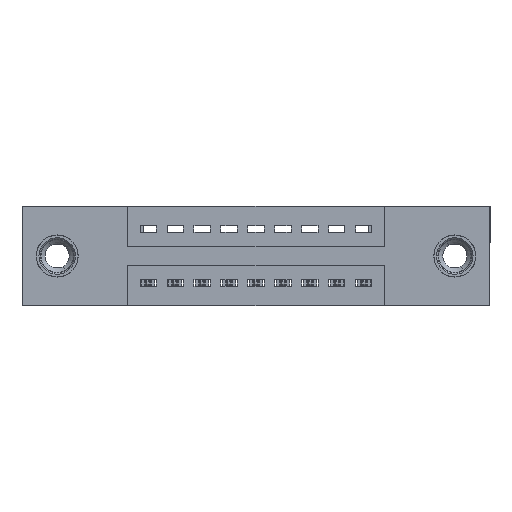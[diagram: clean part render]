
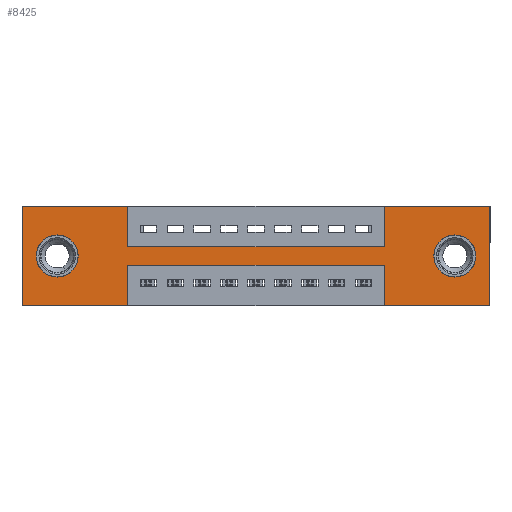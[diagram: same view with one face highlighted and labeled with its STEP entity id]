
A CAD part, front view. The second image highlights one B-rep face of the part: STEP entity #8425.
In plain terms, the highlighted planar face has unit normal (0, -1, 0).
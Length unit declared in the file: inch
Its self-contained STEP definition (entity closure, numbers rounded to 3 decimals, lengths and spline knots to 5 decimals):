
#80 = EDGE_CURVE ( 'NONE', #3752, #586, #3976, .T. ) ;
#113 = EDGE_CURVE ( 'NONE', #8983, #13188, #11638, .T. ) ;
#175 = DIRECTION ( 'NONE',  ( 0., 0., -1. ) ) ;
#392 = DIRECTION ( 'NONE',  ( 0., 1., 0. ) ) ;
#417 = LINE ( 'NONE', #14052, #2769 ) ;
#498 = ORIENTED_EDGE ( 'NONE', *, *, #80, .F. ) ;
#586 = VERTEX_POINT ( 'NONE', #14877 ) ;
#707 = ORIENTED_EDGE ( 'NONE', *, *, #6458, .F. ) ;
#833 = ORIENTED_EDGE ( 'NONE', *, *, #4061, .F. ) ;
#835 = EDGE_CURVE ( 'NONE', #6076, #4176, #8668, .T. ) ;
#995 = VECTOR ( 'NONE', #7859, 39.37008 ) ;
#1015 = VECTOR ( 'NONE', #15629, 39.37008 ) ;
#1167 = VERTEX_POINT ( 'NONE', #13422 ) ;
#1375 = VECTOR ( 'NONE', #2365, 39.37008 ) ;
#1407 = EDGE_CURVE ( 'NONE', #15398, #14669, #15788, .T. ) ;
#1421 = EDGE_CURVE ( 'NONE', #1167, #15398, #10657, .T. ) ;
#1586 = CARTESIAN_POINT ( 'NONE',  ( 0., 0., 0. ) ) ;
#1624 = DIRECTION ( 'NONE',  ( 0., -1., 0. ) ) ;
#1841 = EDGE_CURVE ( 'NONE', #9215, #12019, #5447, .T. ) ;
#1917 = VERTEX_POINT ( 'NONE', #3120 ) ;
#2189 = ORIENTED_EDGE ( 'NONE', *, *, #7108, .F. ) ;
#2365 = DIRECTION ( 'NONE',  ( -1., 0., 0. ) ) ;
#2640 = VECTOR ( 'NONE', #10238, 39.37008 ) ;
#2645 = CARTESIAN_POINT ( 'NONE',  ( 0.3925, 0., -0.37 ) ) ;
#2660 = CARTESIAN_POINT ( 'NONE',  ( 0., 0., -0.37 ) ) ;
#2769 = VECTOR ( 'NONE', #11385, 39.37008 ) ;
#2823 = CARTESIAN_POINT ( 'NONE',  ( 0.13, 0., -0.107 ) ) ;
#2873 = CARTESIAN_POINT ( 'NONE',  ( 1.735, 0., 0. ) ) ;
#2982 = CARTESIAN_POINT ( 'NONE',  ( 1.605, 0., -0.263 ) ) ;
#3120 = CARTESIAN_POINT ( 'NONE',  ( 1.3425, 0., -0.37 ) ) ;
#3184 = CARTESIAN_POINT ( 'NONE',  ( 1.3425, 0., 0. ) ) ;
#3246 = ORIENTED_EDGE ( 'NONE', *, *, #8589, .F. ) ;
#3310 = EDGE_LOOP ( 'NONE', ( #13696, #6005, #3246, #2189, #6740, #5573, #14188, #707, #12571, #498, #7220, #833 ) ) ;
#3475 = EDGE_CURVE ( 'NONE', #12019, #9215, #6502, .T. ) ;
#3740 = VECTOR ( 'NONE', #4452, 39.37008 ) ;
#3752 = VERTEX_POINT ( 'NONE', #6639 ) ;
#3893 = LINE ( 'NONE', #2660, #8349 ) ;
#3976 = LINE ( 'NONE', #1586, #995 ) ;
#4061 = EDGE_CURVE ( 'NONE', #4176, #5098, #3893, .T. ) ;
#4176 = VERTEX_POINT ( 'NONE', #6863 ) ;
#4195 = EDGE_CURVE ( 'NONE', #4606, #6076, #9405, .T. ) ;
#4267 = CARTESIAN_POINT ( 'NONE',  ( 1.605, 0., -0.185 ) ) ;
#4347 = DIRECTION ( 'NONE',  ( 0., 0., -1. ) ) ;
#4418 = DIRECTION ( 'NONE',  ( 0., 1., 0. ) ) ;
#4452 = DIRECTION ( 'NONE',  ( 1., 0., 0. ) ) ;
#4495 = EDGE_CURVE ( 'NONE', #5098, #3752, #7562, .T. ) ;
#4606 = VERTEX_POINT ( 'NONE', #9433 ) ;
#4640 = VECTOR ( 'NONE', #10030, 39.37008 ) ;
#4838 = CARTESIAN_POINT ( 'NONE',  ( 1.735, 0., 0. ) ) ;
#5098 = VERTEX_POINT ( 'NONE', #11167 ) ;
#5101 = AXIS2_PLACEMENT_3D ( 'NONE', #12223, #13770, #7516 ) ;
#5447 = CIRCLE ( 'NONE', #15825, 0.078 ) ;
#5573 = ORIENTED_EDGE ( 'NONE', *, *, #1407, .F. ) ;
#5607 = EDGE_LOOP ( 'NONE', ( #12406, #14906 ) ) ;
#5623 = FACE_BOUND ( 'NONE', #11989, .T. ) ;
#6005 = ORIENTED_EDGE ( 'NONE', *, *, #4195, .F. ) ;
#6076 = VERTEX_POINT ( 'NONE', #10869 ) ;
#6458 = EDGE_CURVE ( 'NONE', #12441, #1167, #15596, .T. ) ;
#6502 = CIRCLE ( 'NONE', #8864, 0.078 ) ;
#6639 = CARTESIAN_POINT ( 'NONE',  ( 0., 0., 0. ) ) ;
#6740 = ORIENTED_EDGE ( 'NONE', *, *, #9463, .F. ) ;
#6856 = ORIENTED_EDGE ( 'NONE', *, *, #10745, .T. ) ;
#6858 = AXIS2_PLACEMENT_3D ( 'NONE', #7820, #1624, #11560 ) ;
#6863 = CARTESIAN_POINT ( 'NONE',  ( 0.3925, 0., -0.37 ) ) ;
#6919 = CARTESIAN_POINT ( 'NONE',  ( 1.735, 0., -0.37 ) ) ;
#7108 = EDGE_CURVE ( 'NONE', #11058, #1917, #13586, .T. ) ;
#7220 = ORIENTED_EDGE ( 'NONE', *, *, #4495, .F. ) ;
#7516 = DIRECTION ( 'NONE',  ( 0., 0., 1. ) ) ;
#7562 = LINE ( 'NONE', #13820, #2640 ) ;
#7614 = DIRECTION ( 'NONE',  ( -1., 0., 0. ) ) ;
#7820 = CARTESIAN_POINT ( 'NONE',  ( 0., 0., -0.37 ) ) ;
#7859 = DIRECTION ( 'NONE',  ( 1., 0., 0. ) ) ;
#8099 = CARTESIAN_POINT ( 'NONE',  ( 1.605, 0., -0.107 ) ) ;
#8181 = DIRECTION ( 'NONE',  ( -1., 0., 0. ) ) ;
#8219 = LINE ( 'NONE', #13157, #13339 ) ;
#8227 = DIRECTION ( 'NONE',  ( 1., 0., 0. ) ) ;
#8349 = VECTOR ( 'NONE', #7614, 39.37008 ) ;
#8425 = ADVANCED_FACE ( 'NONE', ( #10246, #5623, #15209 ), #10408, .T. ) ;
#8440 = CARTESIAN_POINT ( 'NONE',  ( 0.13, 0., -0.263 ) ) ;
#8589 = EDGE_CURVE ( 'NONE', #1917, #4606, #8219, .T. ) ;
#8668 = LINE ( 'NONE', #2645, #4640 ) ;
#8864 = AXIS2_PLACEMENT_3D ( 'NONE', #12421, #14953, #175 ) ;
#8888 = VECTOR ( 'NONE', #8181, 39.37008 ) ;
#8983 = VERTEX_POINT ( 'NONE', #8440 ) ;
#9215 = VERTEX_POINT ( 'NONE', #2982 ) ;
#9405 = LINE ( 'NONE', #14341, #8888 ) ;
#9433 = CARTESIAN_POINT ( 'NONE',  ( 1.3425, 0., -0.22 ) ) ;
#9463 = EDGE_CURVE ( 'NONE', #14669, #11058, #11179, .T. ) ;
#9574 = ORIENTED_EDGE ( 'NONE', *, *, #113, .T. ) ;
#10012 = CIRCLE ( 'NONE', #5101, 0.078 ) ;
#10030 = DIRECTION ( 'NONE',  ( 0., 0., -1. ) ) ;
#10238 = DIRECTION ( 'NONE',  ( 0., 0., 1. ) ) ;
#10246 = FACE_BOUND ( 'NONE', #5607, .T. ) ;
#10286 = DIRECTION ( 'NONE',  ( 0., 0., 1. ) ) ;
#10408 = PLANE ( 'NONE',  #6858 ) ;
#10657 = LINE ( 'NONE', #3184, #1015 ) ;
#10739 = CARTESIAN_POINT ( 'NONE',  ( 0., 0., 0. ) ) ;
#10745 = EDGE_CURVE ( 'NONE', #13188, #8983, #10012, .T. ) ;
#10869 = CARTESIAN_POINT ( 'NONE',  ( 0.3925, 0., -0.22 ) ) ;
#11058 = VERTEX_POINT ( 'NONE', #6919 ) ;
#11167 = CARTESIAN_POINT ( 'NONE',  ( 0., 0., -0.37 ) ) ;
#11179 = LINE ( 'NONE', #4838, #12838 ) ;
#11385 = DIRECTION ( 'NONE',  ( 0., 0., -1. ) ) ;
#11521 = CARTESIAN_POINT ( 'NONE',  ( 0.13, 0., -0.185 ) ) ;
#11560 = DIRECTION ( 'NONE',  ( 0., 0., -1. ) ) ;
#11638 = CIRCLE ( 'NONE', #15009, 0.078 ) ;
#11740 = CARTESIAN_POINT ( 'NONE',  ( 0.3925, 0., -0.15 ) ) ;
#11989 = EDGE_LOOP ( 'NONE', ( #6856, #9574 ) ) ;
#12019 = VERTEX_POINT ( 'NONE', #8099 ) ;
#12172 = CARTESIAN_POINT ( 'NONE',  ( 1.3425, 0., 0. ) ) ;
#12223 = CARTESIAN_POINT ( 'NONE',  ( 0.13, 0., -0.185 ) ) ;
#12406 = ORIENTED_EDGE ( 'NONE', *, *, #3475, .T. ) ;
#12418 = DIRECTION ( 'NONE',  ( 0., 0., 1. ) ) ;
#12421 = CARTESIAN_POINT ( 'NONE',  ( 1.605, 0., -0.185 ) ) ;
#12441 = VERTEX_POINT ( 'NONE', #11740 ) ;
#12571 = ORIENTED_EDGE ( 'NONE', *, *, #12771, .F. ) ;
#12771 = EDGE_CURVE ( 'NONE', #586, #12441, #417, .T. ) ;
#12838 = VECTOR ( 'NONE', #13685, 39.37008 ) ;
#13157 = CARTESIAN_POINT ( 'NONE',  ( 1.3425, 0., -0.37 ) ) ;
#13188 = VERTEX_POINT ( 'NONE', #2823 ) ;
#13339 = VECTOR ( 'NONE', #12418, 39.37008 ) ;
#13422 = CARTESIAN_POINT ( 'NONE',  ( 1.3425, 0., -0.15 ) ) ;
#13504 = CARTESIAN_POINT ( 'NONE',  ( 0., 0., -0.37 ) ) ;
#13586 = LINE ( 'NONE', #13504, #1375 ) ;
#13685 = DIRECTION ( 'NONE',  ( 0., 0., -1. ) ) ;
#13696 = ORIENTED_EDGE ( 'NONE', *, *, #835, .F. ) ;
#13770 = DIRECTION ( 'NONE',  ( 0., 1., 0. ) ) ;
#13820 = CARTESIAN_POINT ( 'NONE',  ( 0., 0., 0. ) ) ;
#14052 = CARTESIAN_POINT ( 'NONE',  ( 0.3925, 0., 0. ) ) ;
#14188 = ORIENTED_EDGE ( 'NONE', *, *, #1421, .F. ) ;
#14341 = CARTESIAN_POINT ( 'NONE',  ( 0.3925, 0., -0.22 ) ) ;
#14669 = VERTEX_POINT ( 'NONE', #2873 ) ;
#14877 = CARTESIAN_POINT ( 'NONE',  ( 0.3925, 0., 0. ) ) ;
#14906 = ORIENTED_EDGE ( 'NONE', *, *, #1841, .T. ) ;
#14953 = DIRECTION ( 'NONE',  ( 0., 1., 0. ) ) ;
#15009 = AXIS2_PLACEMENT_3D ( 'NONE', #11521, #392, #10286 ) ;
#15209 = FACE_OUTER_BOUND ( 'NONE', #3310, .T. ) ;
#15294 = VECTOR ( 'NONE', #8227, 39.37008 ) ;
#15398 = VERTEX_POINT ( 'NONE', #12172 ) ;
#15596 = LINE ( 'NONE', #15677, #3740 ) ;
#15629 = DIRECTION ( 'NONE',  ( 0., 0., 1. ) ) ;
#15677 = CARTESIAN_POINT ( 'NONE',  ( 0.3925, 0., -0.15 ) ) ;
#15788 = LINE ( 'NONE', #10739, #15294 ) ;
#15825 = AXIS2_PLACEMENT_3D ( 'NONE', #4267, #4418, #4347 ) ;
